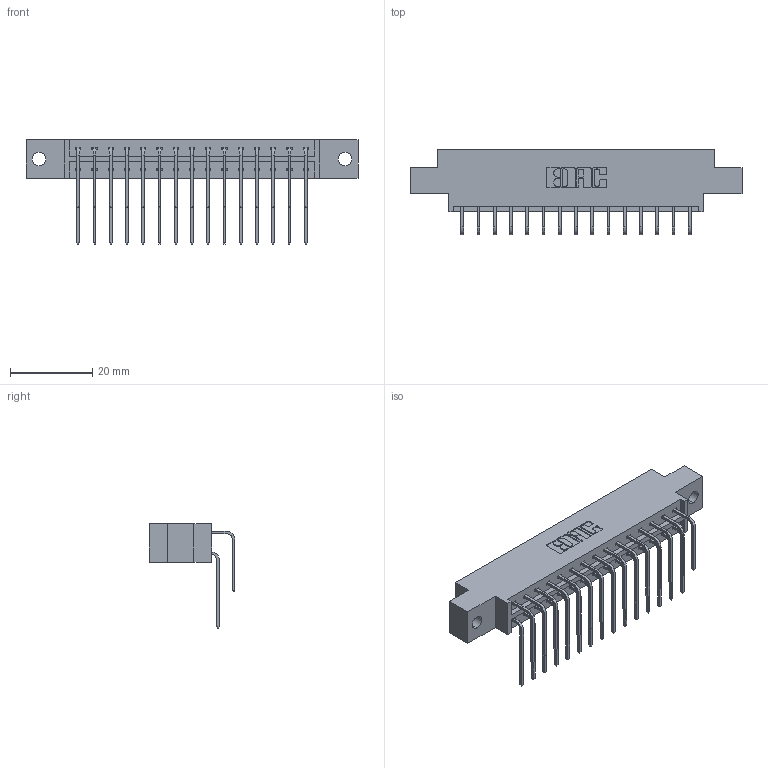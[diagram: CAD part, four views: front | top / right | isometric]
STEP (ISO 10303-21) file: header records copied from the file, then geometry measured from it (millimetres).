
FILE_DESCRIPTION (( 'STEP AP203' ), '1' );
FILE_NAME ('833-030-559-802.STEP', '2020-06-02T14:36:31', ( '' ), ( '' ), 'SwSTEP 2.0', 'SolidWorks 2020', '' );
FILE_SCHEMA (( 'CONFIG_CONTROL_DESIGN' ));
Length unit declared in the file: inch
Products named in the file (4): 345-292-001_558 559 Tail - 1; 833-030-559-802; 833 Part_Offset - .128 Dia; 345-292-001_559 Tail - 2
Assembly tree (31 placements, depth 2):
  833-030-559-802
    833 Part_Offset - .128 Dia
    345-292-001_558 559 Tail - 1  x15
    345-292-001_559 Tail - 2  x15
Bounding box: 80.98 x 20.9 x 25.53 mm (x, y, z)
Volume: 7923.2 mm3; surface area: 9886.6 mm2
Topology: 31 solids, 31 shells, 1738 faces, 5153 edges, 3394 vertices
Faces by surface type: plane 1214, cylinder 524
Entity records: 15061 total; most frequent: CARTESIAN_POINT 2581, ORIENTED_EDGE 2466, DIRECTION 2233, EDGE_CURVE 1233, LINE 1065, VECTOR 1065, VERTEX_POINT 818, AXIS2_PLACEMENT_3D 584
